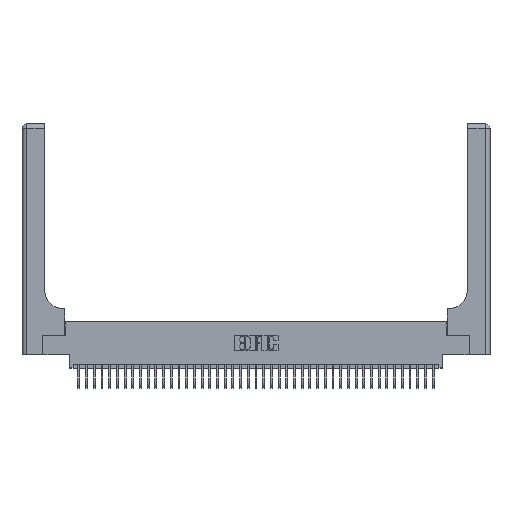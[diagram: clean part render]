
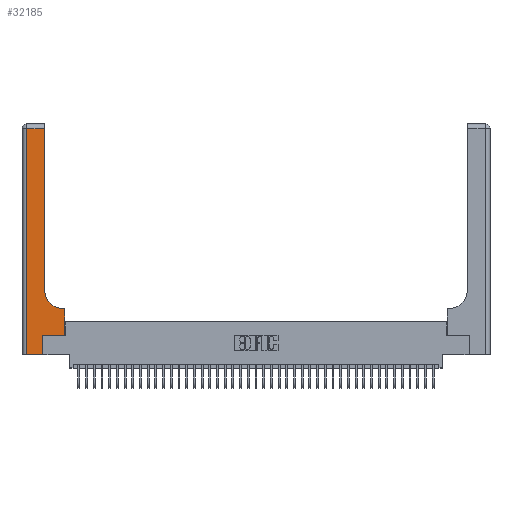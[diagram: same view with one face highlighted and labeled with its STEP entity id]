
A CAD part, top view. The second image highlights one B-rep face of the part: STEP entity #32185.
In plain terms, the highlighted planar face has unit normal (0, 0, 1).
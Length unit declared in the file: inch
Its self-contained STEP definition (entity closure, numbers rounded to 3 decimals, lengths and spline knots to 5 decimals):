
#513 = VERTEX_POINT ( 'NONE', #13901 ) ;
#682 = DIRECTION ( 'NONE',  ( 0., 0., -1. ) ) ;
#1101 = EDGE_CURVE ( 'NONE', #513, #2368, #28488, .T. ) ;
#1108 = EDGE_CURVE ( 'NONE', #3281, #24176, #29521, .T. ) ;
#2005 = CARTESIAN_POINT ( 'NONE',  ( 0.2915, 2.94, 0.37 ) ) ;
#2136 = ORIENTED_EDGE ( 'NONE', *, *, #1101, .T. ) ;
#2368 = VERTEX_POINT ( 'NONE', #21479 ) ;
#2389 = DIRECTION ( 'NONE',  ( 1., 0., 0. ) ) ;
#2539 = DIRECTION ( 'NONE',  ( -1., 0., 0. ) ) ;
#2543 = AXIS2_PLACEMENT_3D ( 'NONE', #3876, #682, #33820 ) ;
#2824 = ORIENTED_EDGE ( 'NONE', *, *, #18973, .T. ) ;
#2949 = LINE ( 'NONE', #5635, #34468 ) ;
#3033 = VERTEX_POINT ( 'NONE', #42852 ) ;
#3098 = FACE_OUTER_BOUND ( 'NONE', #38893, .T. ) ;
#3281 = VERTEX_POINT ( 'NONE', #11458 ) ;
#3876 = CARTESIAN_POINT ( 'NONE',  ( 0., 3., 0.37 ) ) ;
#4244 = ORIENTED_EDGE ( 'NONE', *, *, #14442, .T. ) ;
#4531 = EDGE_CURVE ( 'NONE', #7699, #40877, #41284, .T. ) ;
#4611 = ORIENTED_EDGE ( 'NONE', *, *, #4531, .T. ) ;
#5271 = EDGE_CURVE ( 'NONE', #2368, #31796, #30480, .T. ) ;
#5635 = CARTESIAN_POINT ( 'NONE',  ( 0., 2.94, 0.37 ) ) ;
#7076 = VECTOR ( 'NONE', #10676, 39.37008 ) ;
#7637 = ORIENTED_EDGE ( 'NONE', *, *, #13120, .T. ) ;
#7699 = VERTEX_POINT ( 'NONE', #14195 ) ;
#8160 = CARTESIAN_POINT ( 'NONE',  ( 0.5585, 0.25, 0.37 ) ) ;
#8353 = VECTOR ( 'NONE', #19033, 39.37008 ) ;
#9239 = CARTESIAN_POINT ( 'NONE',  ( 0.2915, 0.6, 0.37 ) ) ;
#9799 = LINE ( 'NONE', #8160, #20809 ) ;
#10676 = DIRECTION ( 'NONE',  ( 1., 0., 0. ) ) ;
#10699 = VECTOR ( 'NONE', #19677, 39.37008 ) ;
#11458 = CARTESIAN_POINT ( 'NONE',  ( 0.2915, 0.85, 0.37 ) ) ;
#11651 = VECTOR ( 'NONE', #2389, 39.37008 ) ;
#11718 = DIRECTION ( 'NONE',  ( 0., 0., -1. ) ) ;
#12740 = CARTESIAN_POINT ( 'NONE',  ( 0.5415, 0.6, 0.37 ) ) ;
#12801 = CARTESIAN_POINT ( 'NONE',  ( 0.269, 0., 0.37 ) ) ;
#13120 = EDGE_CURVE ( 'NONE', #28608, #3033, #40177, .T. ) ;
#13901 = CARTESIAN_POINT ( 'NONE',  ( 0.269, 0., 0.37 ) ) ;
#14195 = CARTESIAN_POINT ( 'NONE',  ( 0.5585, 0.6, 0.37 ) ) ;
#14442 = EDGE_CURVE ( 'NONE', #31796, #7699, #9799, .T. ) ;
#15052 = DIRECTION ( 'NONE',  ( 0., 1., 0. ) ) ;
#17007 = ORIENTED_EDGE ( 'NONE', *, *, #1108, .T. ) ;
#18887 = ORIENTED_EDGE ( 'NONE', *, *, #28657, .T. ) ;
#18973 = EDGE_CURVE ( 'NONE', #24176, #28608, #2949, .T. ) ;
#19033 = DIRECTION ( 'NONE',  ( 0., -1., 0. ) ) ;
#19677 = DIRECTION ( 'NONE',  ( 0., 1., 0. ) ) ;
#20180 = CIRCLE ( 'NONE', #41355, 0.25 ) ;
#20809 = VECTOR ( 'NONE', #15052, 39.37008 ) ;
#21479 = CARTESIAN_POINT ( 'NONE',  ( 0.269, 0.25, 0.37 ) ) ;
#21712 = VECTOR ( 'NONE', #30927, 39.37008 ) ;
#23556 = ORIENTED_EDGE ( 'NONE', *, *, #5271, .T. ) ;
#24176 = VERTEX_POINT ( 'NONE', #2005 ) ;
#26601 = CARTESIAN_POINT ( 'NONE',  ( 0., 0., 0.37 ) ) ;
#28303 = EDGE_CURVE ( 'NONE', #40877, #3281, #20180, .T. ) ;
#28488 = LINE ( 'NONE', #12801, #21712 ) ;
#28608 = VERTEX_POINT ( 'NONE', #29532 ) ;
#28657 = EDGE_CURVE ( 'NONE', #3033, #513, #36872, .T. ) ;
#28976 = CARTESIAN_POINT ( 'NONE',  ( 0.269, 0.25, 0.37 ) ) ;
#29521 = LINE ( 'NONE', #32821, #10699 ) ;
#29532 = CARTESIAN_POINT ( 'NONE',  ( 0.06, 2.94, 0.37 ) ) ;
#29883 = DIRECTION ( 'NONE',  ( -1., 0., 0. ) ) ;
#30480 = LINE ( 'NONE', #28976, #11651 ) ;
#30604 = PLANE ( 'NONE',  #2543 ) ;
#30927 = DIRECTION ( 'NONE',  ( 0., 1., 0. ) ) ;
#31796 = VERTEX_POINT ( 'NONE', #37789 ) ;
#32185 = ADVANCED_FACE ( 'NONE', ( #3098 ), #30604, .F. ) ;
#32821 = CARTESIAN_POINT ( 'NONE',  ( 0.2915, 3., 0.37 ) ) ;
#33820 = DIRECTION ( 'NONE',  ( -1., 0., 0. ) ) ;
#34468 = VECTOR ( 'NONE', #29883, 39.37008 ) ;
#35112 = DIRECTION ( 'NONE',  ( 1., 0., 0. ) ) ;
#36872 = LINE ( 'NONE', #26601, #7076 ) ;
#37277 = ORIENTED_EDGE ( 'NONE', *, *, #28303, .T. ) ;
#37789 = CARTESIAN_POINT ( 'NONE',  ( 0.5585, 0.25, 0.37 ) ) ;
#38316 = CARTESIAN_POINT ( 'NONE',  ( 0.5415, 0.85, 0.37 ) ) ;
#38893 = EDGE_LOOP ( 'NONE', ( #17007, #2824, #7637, #18887, #2136, #23556, #4244, #4611, #37277 ) ) ;
#39194 = VECTOR ( 'NONE', #2539, 39.37008 ) ;
#39291 = CARTESIAN_POINT ( 'NONE',  ( 0.06, 3., 0.37 ) ) ;
#40177 = LINE ( 'NONE', #39291, #8353 ) ;
#40877 = VERTEX_POINT ( 'NONE', #12740 ) ;
#41284 = LINE ( 'NONE', #9239, #39194 ) ;
#41355 = AXIS2_PLACEMENT_3D ( 'NONE', #38316, #11718, #35112 ) ;
#42852 = CARTESIAN_POINT ( 'NONE',  ( 0.06, 0., 0.37 ) ) ;
